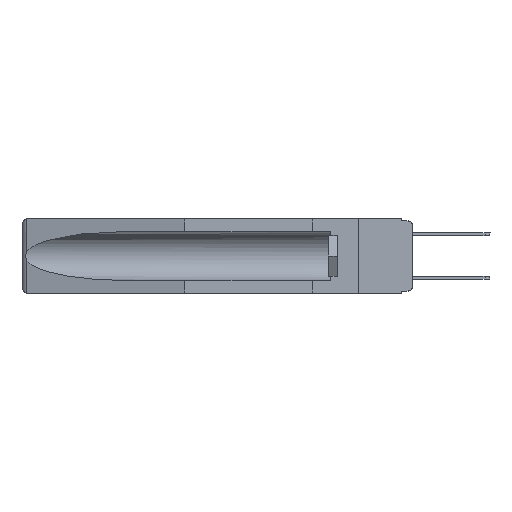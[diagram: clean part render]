
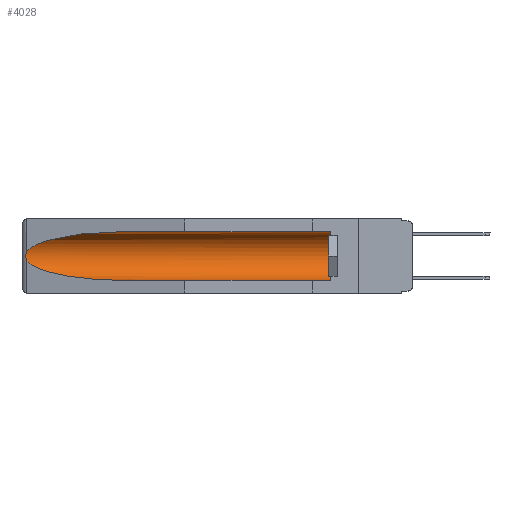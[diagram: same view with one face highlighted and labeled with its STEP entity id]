
A CAD part, left-side view. The second image highlights one B-rep face of the part: STEP entity #4028.
In plain terms, the highlighted cylindrical face has radius 2.857 mm (diameter 5.715 mm), a partial arc.
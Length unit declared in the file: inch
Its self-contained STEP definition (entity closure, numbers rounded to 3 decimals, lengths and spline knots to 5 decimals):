
#97 = CARTESIAN_POINT ( 'NONE',  ( 0.155, 0.126, -0.1715 ) ) ;
#1125 = ORIENTED_EDGE ( 'NONE', *, *, #12420, .T. ) ;
#1459 = EDGE_CURVE ( 'NONE', #16445, #17639, #7802, .T. ) ;
#2465 = CYLINDRICAL_SURFACE ( 'NONE', #2785, 0.1125 ) ;
#2785 = AXIS2_PLACEMENT_3D ( 'NONE', #9050, #15637, #17038 ) ;
#2883 = CARTESIAN_POINT ( 'NONE',  ( 0.25451, 1.48313, -0.24835 ) ) ;
#3015 = CARTESIAN_POINT ( 'NONE',  ( 0.21114, 1.30732, -0.059 ) ) ;
#4028 = ADVANCED_FACE ( 'NONE', ( #15315 ), #2465, .F. ) ;
#4253 = CARTESIAN_POINT ( 'NONE',  ( 0.26537, 1.52718, -0.14972 ) ) ;
#4491 = CARTESIAN_POINT ( 'NONE',  ( 0.26537, 1.52718, -0.19328 ) ) ;
#4537 = CARTESIAN_POINT ( 'NONE',  ( 0.26537, 1.52718, -0.14972 ) ) ;
#4849 = ORIENTED_EDGE ( 'NONE', *, *, #1459, .F. ) ;
#5105 = EDGE_LOOP ( 'NONE', ( #21239, #13240, #1125, #4849, #15048, #8732 ) ) ;
#5405 = VECTOR ( 'NONE', #10264, 39.37008 ) ;
#5648 = CARTESIAN_POINT ( 'NONE',  ( 0.2675, 1.53308, -0.16763 ) ) ;
#6014 = CARTESIAN_POINT ( 'NONE',  ( 0.155, 0.126, -0.284 ) ) ;
#6367 = B_SPLINE_CURVE_WITH_KNOTS ( 'NONE', 3,
 ( #4253, #15703, #20606, #12375, #5648, #18991, #17446, #18859, #7602, #19196 ),
 .UNSPECIFIED., .F., .F.,
 ( 4, 2, 2, 2, 4 ),
 ( 0., 0.00029, 0.00058, 0.00087, 0.00117 ),
 .UNSPECIFIED. ) ;
#6670 = DIRECTION ( 'NONE',  ( 0., -1., 0. ) ) ;
#7602 = CARTESIAN_POINT ( 'NONE',  ( 0.26597, 1.5296, -0.19026 ) ) ;
#7802 = LINE ( 'NONE', #16019, #13410 ) ;
#8428 = CARTESIAN_POINT ( 'NONE',  ( 0.155, 1.07973, -0.059 ) ) ;
#8732 = ORIENTED_EDGE ( 'NONE', *, *, #14396, .T. ) ;
#9050 = CARTESIAN_POINT ( 'NONE',  ( 0.155, -0.30754, -0.1715 ) ) ;
#9458 = CARTESIAN_POINT ( 'NONE',  ( 0.155, 1.07973, -0.284 ) ) ;
#9604 = CARTESIAN_POINT ( 'NONE',  ( 0.26537, 1.52718, -0.14972 ) ) ;
#9636 = CIRCLE ( 'NONE', #15156, 0.1125 ) ;
#9678 = CARTESIAN_POINT ( 'NONE',  ( 0.21114, 1.30732, -0.284 ) ) ;
#10264 = DIRECTION ( 'NONE',  ( 0., 1., 0. ) ) ;
#11509 = CARTESIAN_POINT ( 'NONE',  ( 0.155, 0.126, -0.059 ) ) ;
#11702 = VERTEX_POINT ( 'NONE', #4537 ) ;
#12375 = CARTESIAN_POINT ( 'NONE',  ( 0.2673, 1.5327, -0.16383 ) ) ;
#12420 = EDGE_CURVE ( 'NONE', #19009, #17639, #18006, .T. ) ;
#12434 = CARTESIAN_POINT ( 'NONE',  ( 0.155, 1.07973, -0.059 ) ) ;
#13116 = EDGE_CURVE ( 'NONE', #16445, #14004, #9636, .T. ) ;
#13240 = ORIENTED_EDGE ( 'NONE', *, *, #17857, .T. ) ;
#13289 = DIRECTION ( 'NONE',  ( 0., 0., 1. ) ) ;
#13410 = VECTOR ( 'NONE', #21358, 39.37008 ) ;
#14004 = VERTEX_POINT ( 'NONE', #11509 ) ;
#14396 = EDGE_CURVE ( 'NONE', #14004, #19423, #16545, .T. ) ;
#15048 = ORIENTED_EDGE ( 'NONE', *, *, #13116, .T. ) ;
#15156 = AXIS2_PLACEMENT_3D ( 'NONE', #97, #6670, #13289 ) ;
#15315 = FACE_OUTER_BOUND ( 'NONE', #5105, .T. ) ;
#15637 = DIRECTION ( 'NONE',  ( 0., 1., 0. ) ) ;
#15703 = CARTESIAN_POINT ( 'NONE',  ( 0.26597, 1.52961, -0.15275 ) ) ;
#15878 = CARTESIAN_POINT ( 'NONE',  ( 0.25451, 1.48313, -0.09465 ) ) ;
#16019 = CARTESIAN_POINT ( 'NONE',  ( 0.155, -0.30754, -0.284 ) ) ;
#16445 = VERTEX_POINT ( 'NONE', #6014 ) ;
#16545 = LINE ( 'NONE', #18287, #5405 ) ;
#16792 = CARTESIAN_POINT ( 'NONE',  ( 0.155, 1.07973, -0.284 ) ) ;
#17038 = DIRECTION ( 'NONE',  ( 0., 0., 1. ) ) ;
#17446 = CARTESIAN_POINT ( 'NONE',  ( 0.2673, 1.53269, -0.17917 ) ) ;
#17585 = EDGE_CURVE ( 'NONE', #19423, #11702, #18118, .T. ) ;
#17639 = VERTEX_POINT ( 'NONE', #16792 ) ;
#17857 = EDGE_CURVE ( 'NONE', #11702, #19009, #6367, .T. ) ;
#18006 =( BOUNDED_CURVE ( )  B_SPLINE_CURVE ( 3, ( #4491, #2883, #9678, #9458 ),
 .UNSPECIFIED., .F., .T. ) 
 B_SPLINE_CURVE_WITH_KNOTS ( ( 4, 4 ),
 ( 0.1948, 1.5708 ),
 .UNSPECIFIED. ) 
 CURVE ( )  GEOMETRIC_REPRESENTATION_ITEM ( )  RATIONAL_B_SPLINE_CURVE ( ( 1., 0.848, 0.848, 1. ) ) 
 REPRESENTATION_ITEM ( '' )  );
#18118 =( BOUNDED_CURVE ( )  B_SPLINE_CURVE ( 3, ( #12434, #3015, #15878, #9604 ),
 .UNSPECIFIED., .F., .T. ) 
 B_SPLINE_CURVE_WITH_KNOTS ( ( 4, 4 ),
 ( 4.71239, 6.08839 ),
 .UNSPECIFIED. ) 
 CURVE ( )  GEOMETRIC_REPRESENTATION_ITEM ( )  RATIONAL_B_SPLINE_CURVE ( ( 1., 0.848, 0.848, 1. ) ) 
 REPRESENTATION_ITEM ( '' )  );
#18134 = CARTESIAN_POINT ( 'NONE',  ( 0.26537, 1.52718, -0.19328 ) ) ;
#18287 = CARTESIAN_POINT ( 'NONE',  ( 0.155, -0.30754, -0.059 ) ) ;
#18859 = CARTESIAN_POINT ( 'NONE',  ( 0.26655, 1.53094, -0.18657 ) ) ;
#18991 = CARTESIAN_POINT ( 'NONE',  ( 0.2675, 1.53308, -0.17534 ) ) ;
#19009 = VERTEX_POINT ( 'NONE', #18134 ) ;
#19196 = CARTESIAN_POINT ( 'NONE',  ( 0.26537, 1.52718, -0.19328 ) ) ;
#19423 = VERTEX_POINT ( 'NONE', #8428 ) ;
#20606 = CARTESIAN_POINT ( 'NONE',  ( 0.26654, 1.53092, -0.15636 ) ) ;
#21239 = ORIENTED_EDGE ( 'NONE', *, *, #17585, .T. ) ;
#21358 = DIRECTION ( 'NONE',  ( 0., 1., 0. ) ) ;
